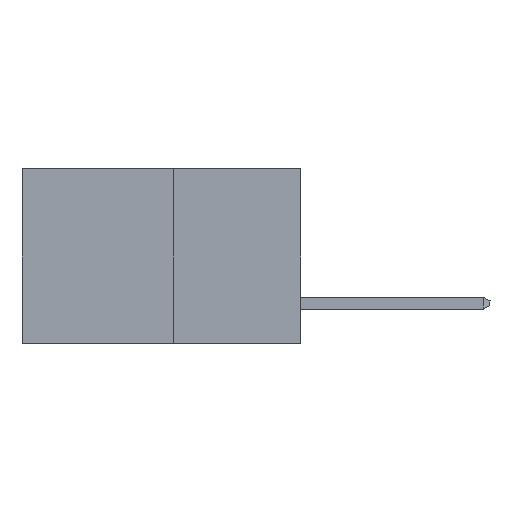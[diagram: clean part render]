
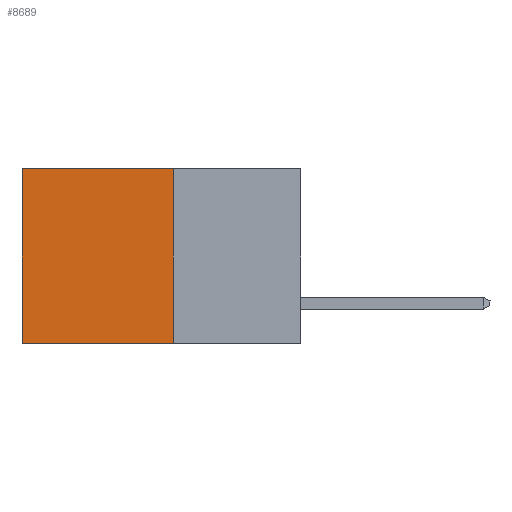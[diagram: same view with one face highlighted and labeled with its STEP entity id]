
A CAD part, left-side view. The second image highlights one B-rep face of the part: STEP entity #8689.
In plain terms, the highlighted planar face has unit normal (-1, 0, 0).
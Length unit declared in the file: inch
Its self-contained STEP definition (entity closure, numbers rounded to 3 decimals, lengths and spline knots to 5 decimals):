
#148 = CARTESIAN_POINT ( 'NONE',  ( 0.277, 0.27, -0.37 ) ) ;
#320 = AXIS2_PLACEMENT_3D ( 'NONE', #25149, #3476, #25686 ) ;
#454 = CARTESIAN_POINT ( 'NONE',  ( 0.277, 0.27, 0. ) ) ;
#788 = EDGE_LOOP ( 'NONE', ( #14751, #32365, #4539, #26686 ) ) ;
#1255 = CARTESIAN_POINT ( 'NONE',  ( 0.277, 0.59, -0.37 ) ) ;
#3476 = DIRECTION ( 'NONE',  ( 1., 0., 0. ) ) ;
#3995 = FACE_OUTER_BOUND ( 'NONE', #788, .T. ) ;
#4539 = ORIENTED_EDGE ( 'NONE', *, *, #21115, .F. ) ;
#4858 = VERTEX_POINT ( 'NONE', #26638 ) ;
#5838 = VECTOR ( 'NONE', #12251, 39.37008 ) ;
#6683 = LINE ( 'NONE', #30956, #5838 ) ;
#7629 = EDGE_CURVE ( 'NONE', #25936, #30967, #25617, .T. ) ;
#8311 = DIRECTION ( 'NONE',  ( 0., 0., -1. ) ) ;
#8381 = CARTESIAN_POINT ( 'NONE',  ( 0.277, 0.59, -0.37 ) ) ;
#8689 = ADVANCED_FACE ( 'NONE', ( #3995 ), #24674, .F. ) ;
#12251 = DIRECTION ( 'NONE',  ( 0., 1., 0. ) ) ;
#14751 = ORIENTED_EDGE ( 'NONE', *, *, #7629, .T. ) ;
#15703 = LINE ( 'NONE', #148, #23616 ) ;
#16310 = DIRECTION ( 'NONE',  ( 0., 1., 0. ) ) ;
#16998 = EDGE_CURVE ( 'NONE', #24893, #25936, #22328, .T. ) ;
#17569 = CARTESIAN_POINT ( 'NONE',  ( 0.277, 0.27, 0. ) ) ;
#17723 = VECTOR ( 'NONE', #8311, 39.37008 ) ;
#21115 = EDGE_CURVE ( 'NONE', #24893, #4858, #15703, .T. ) ;
#21487 = VECTOR ( 'NONE', #16310, 39.37008 ) ;
#22328 = LINE ( 'NONE', #454, #21487 ) ;
#23616 = VECTOR ( 'NONE', #23992, 39.37008 ) ;
#23992 = DIRECTION ( 'NONE',  ( 0., 0., -1. ) ) ;
#24674 = PLANE ( 'NONE',  #320 ) ;
#24893 = VERTEX_POINT ( 'NONE', #17569 ) ;
#25149 = CARTESIAN_POINT ( 'NONE',  ( 0.277, 0.27, -0.37 ) ) ;
#25617 = LINE ( 'NONE', #8381, #17723 ) ;
#25686 = DIRECTION ( 'NONE',  ( 0., 0., -1. ) ) ;
#25936 = VERTEX_POINT ( 'NONE', #31856 ) ;
#26638 = CARTESIAN_POINT ( 'NONE',  ( 0.277, 0.27, -0.37 ) ) ;
#26686 = ORIENTED_EDGE ( 'NONE', *, *, #16998, .T. ) ;
#30956 = CARTESIAN_POINT ( 'NONE',  ( 0.277, 0.27, -0.37 ) ) ;
#30967 = VERTEX_POINT ( 'NONE', #1255 ) ;
#31856 = CARTESIAN_POINT ( 'NONE',  ( 0.277, 0.59, 0. ) ) ;
#32365 = ORIENTED_EDGE ( 'NONE', *, *, #34154, .F. ) ;
#34154 = EDGE_CURVE ( 'NONE', #4858, #30967, #6683, .T. ) ;
